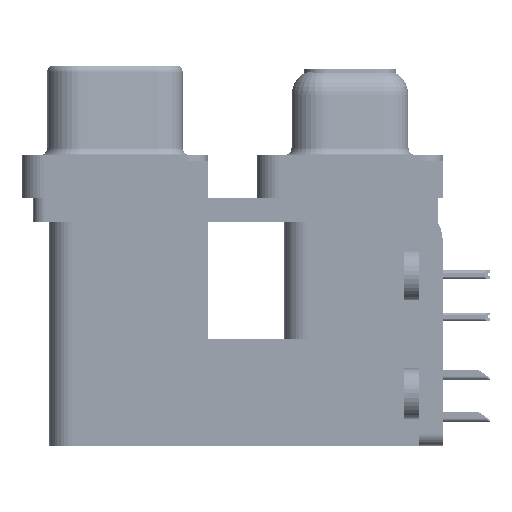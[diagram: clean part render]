
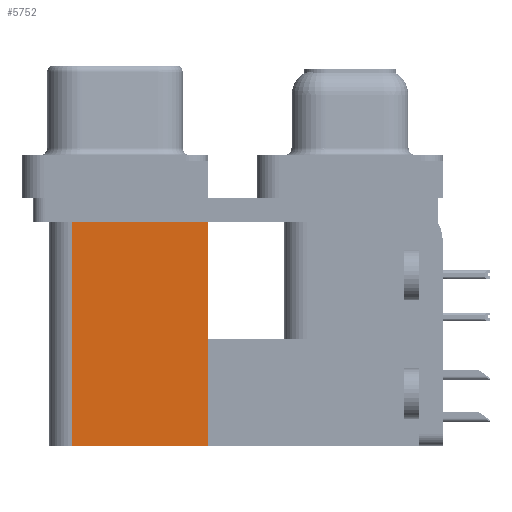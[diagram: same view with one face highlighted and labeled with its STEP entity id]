
A CAD part, left-side view. The second image highlights one B-rep face of the part: STEP entity #5752.
In plain terms, the highlighted planar face has unit normal (-1, 0, 0).
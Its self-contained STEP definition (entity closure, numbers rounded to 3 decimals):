
#1119 = DIRECTION ( 'NONE',  ( 0., 1., 0. ) ) ;
#2483 = DIRECTION ( 'NONE',  ( 1., 0., 0. ) ) ;
#4426 = LINE ( 'NONE', #40673, #46848 ) ;
#5752 = ADVANCED_FACE ( 'NONE', ( #37594 ), #51481, .F. ) ;
#8951 = ORIENTED_EDGE ( 'NONE', *, *, #45499, .F. ) ;
#9468 = EDGE_CURVE ( 'NONE', #26872, #27025, #10081, .T. ) ;
#10081 = LINE ( 'NONE', #45166, #40601 ) ;
#10116 = CARTESIAN_POINT ( 'NONE',  ( 3.7, 9.6, -2.5 ) ) ;
#10604 = VERTEX_POINT ( 'NONE', #31942 ) ;
#10653 = CARTESIAN_POINT ( 'NONE',  ( 3.7, 18.8, -19.2 ) ) ;
#11487 = VECTOR ( 'NONE', #1119, 1000. ) ;
#12382 = VERTEX_POINT ( 'NONE', #18834 ) ;
#13691 = EDGE_CURVE ( 'NONE', #27025, #12382, #31321, .T. ) ;
#14005 = DIRECTION ( 'NONE',  ( 0., 1., 0. ) ) ;
#16606 = ORIENTED_EDGE ( 'NONE', *, *, #19857, .F. ) ;
#18834 = CARTESIAN_POINT ( 'NONE',  ( 3.7, 18.8, -2.5 ) ) ;
#19857 = EDGE_CURVE ( 'NONE', #26872, #10604, #4426, .T. ) ;
#23349 = EDGE_LOOP ( 'NONE', ( #57257, #8951, #16606, #56063 ) ) ;
#25378 = CARTESIAN_POINT ( 'NONE',  ( 3.7, 9.6, -19.2 ) ) ;
#26872 = VERTEX_POINT ( 'NONE', #25378 ) ;
#26881 = VECTOR ( 'NONE', #55297, 1000. ) ;
#27025 = VERTEX_POINT ( 'NONE', #31455 ) ;
#29179 = CARTESIAN_POINT ( 'NONE',  ( 3.7, 9.6, -19.2 ) ) ;
#29452 = DIRECTION ( 'NONE',  ( 0., 0., -1. ) ) ;
#31321 = LINE ( 'NONE', #10116, #11487 ) ;
#31455 = CARTESIAN_POINT ( 'NONE',  ( 3.7, 9.6, -2.5 ) ) ;
#31942 = CARTESIAN_POINT ( 'NONE',  ( 3.7, 18.8, -19.2 ) ) ;
#37594 = FACE_OUTER_BOUND ( 'NONE', #23349, .T. ) ;
#40601 = VECTOR ( 'NONE', #45447, 1000. ) ;
#40673 = CARTESIAN_POINT ( 'NONE',  ( 3.7, 9.6, -19.2 ) ) ;
#45166 = CARTESIAN_POINT ( 'NONE',  ( 3.7, 9.6, -19.2 ) ) ;
#45447 = DIRECTION ( 'NONE',  ( 0., 0., 1. ) ) ;
#45499 = EDGE_CURVE ( 'NONE', #10604, #12382, #50392, .T. ) ;
#46484 = AXIS2_PLACEMENT_3D ( 'NONE', #29179, #2483, #29452 ) ;
#46848 = VECTOR ( 'NONE', #14005, 1000. ) ;
#50392 = LINE ( 'NONE', #10653, #26881 ) ;
#51481 = PLANE ( 'NONE',  #46484 ) ;
#55297 = DIRECTION ( 'NONE',  ( 0., 0., 1. ) ) ;
#56063 = ORIENTED_EDGE ( 'NONE', *, *, #9468, .T. ) ;
#57257 = ORIENTED_EDGE ( 'NONE', *, *, #13691, .T. ) ;
